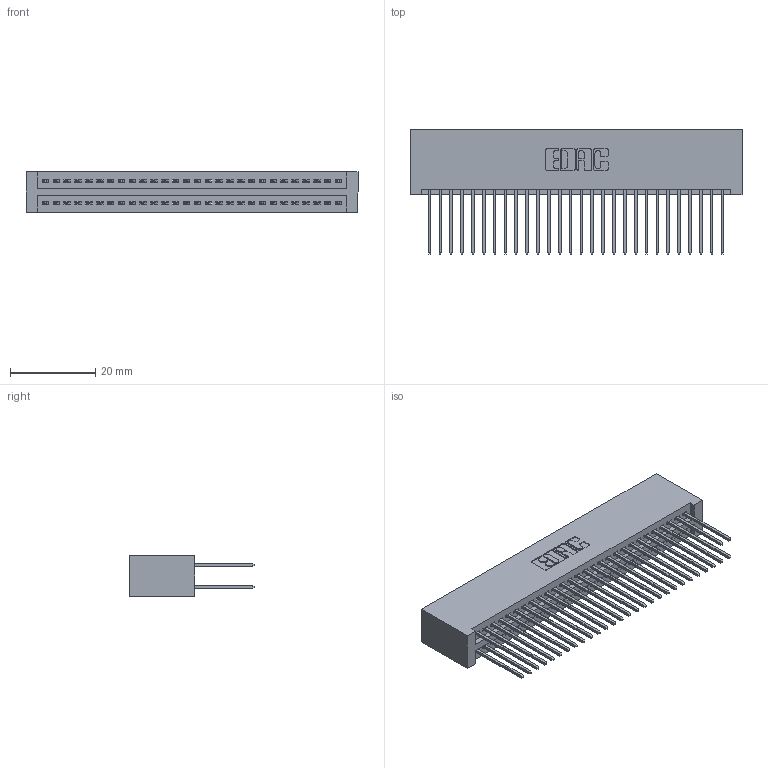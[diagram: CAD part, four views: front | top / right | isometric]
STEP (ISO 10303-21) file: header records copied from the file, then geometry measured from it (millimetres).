
FILE_DESCRIPTION (( 'STEP AP203' ), '1' );
FILE_NAME ('345-056-540-201.STEP', '2019-10-29T21:33:03', ( '' ), ( '' ), 'SwSTEP 2.0', 'SolidWorks 2016', '' );
FILE_SCHEMA (( 'CONFIG_CONTROL_DESIGN' ));
Length unit declared in the file: inch
Products named in the file (3): 345-292-001_345-293-140; 345-056-540-201; 345 Part_No Mounting Lugs
Assembly tree (57 placements, depth 2):
  345-056-540-201
    345 Part_No Mounting Lugs
    345-292-001_345-293-140  x56
Bounding box: 77.72 x 29.13 x 9.4 mm (x, y, z)
Volume: 8248.4 mm3; surface area: 13209.6 mm2
Topology: 57 solids, 57 shells, 2918 faces, 8661 edges, 5698 vertices
Faces by surface type: plane 1924, cylinder 994
Entity records: 23595 total; most frequent: CARTESIAN_POINT 3968, ORIENTED_EDGE 3902, DIRECTION 3511, EDGE_CURVE 1951, LINE 1715, VECTOR 1715, VERTEX_POINT 1298, AXIS2_PLACEMENT_3D 898
